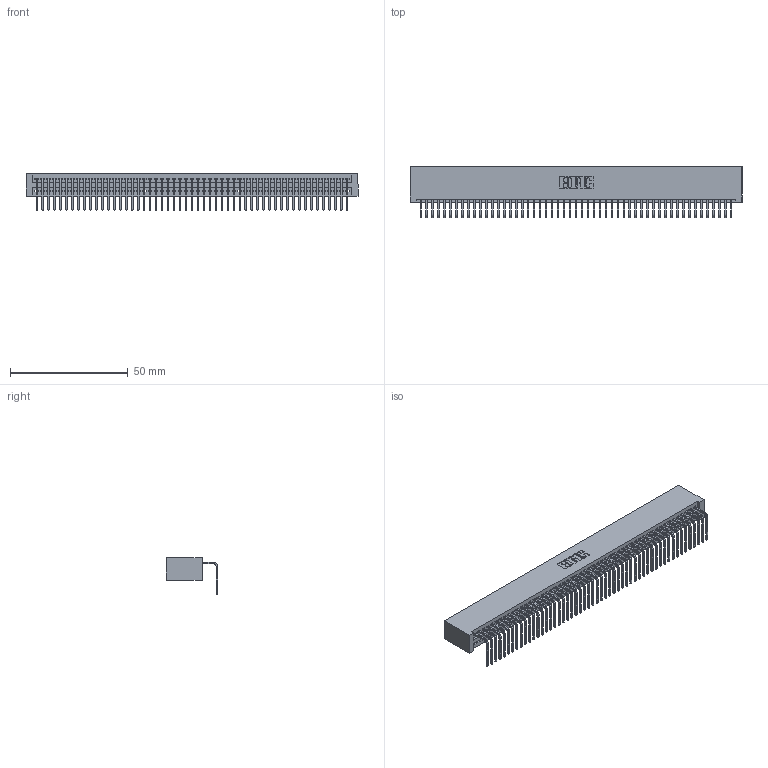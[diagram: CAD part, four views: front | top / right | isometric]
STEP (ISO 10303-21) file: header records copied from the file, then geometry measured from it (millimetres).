
FILE_DESCRIPTION (( 'STEP AP203' ), '1' );
FILE_NAME ('395-053-558-101.STEP', '2019-10-11T14:19:57', ( '' ), ( '' ), 'SwSTEP 2.0', 'SolidWorks 2016', '' );
FILE_SCHEMA (( 'CONFIG_CONTROL_DESIGN' ));
Length unit declared in the file: inch
Products named in the file (3): 395-053-558-101; 345 Part_No Mounting Lugs; 345-292-001_558 Tail - 2
Assembly tree (54 placements, depth 2):
  395-053-558-101
    345 Part_No Mounting Lugs
    345-292-001_558 Tail - 2  x53
Bounding box: 141.22 x 21.83 x 15.37 mm (x, y, z)
Volume: 14264.7 mm3; surface area: 20333.7 mm2
Topology: 54 solids, 54 shells, 3298 faces, 9963 edges, 6570 vertices
Faces by surface type: plane 2302, cylinder 996
Entity records: 38215 total; most frequent: CARTESIAN_POINT 6627, ORIENTED_EDGE 6614, DIRECTION 5765, EDGE_CURVE 3307, LINE 2971, VECTOR 2971, VERTEX_POINT 2202, AXIS2_PLACEMENT_3D 1397
